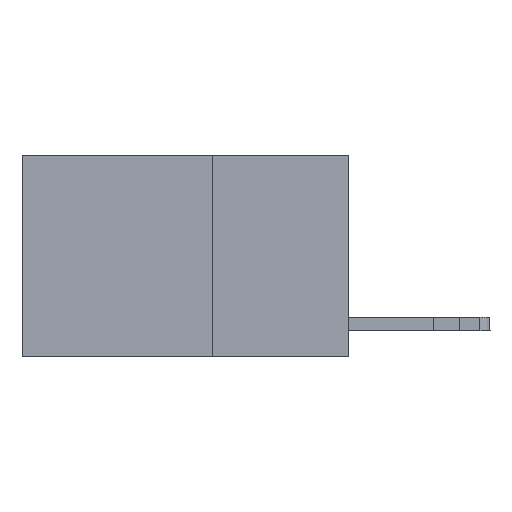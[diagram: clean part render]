
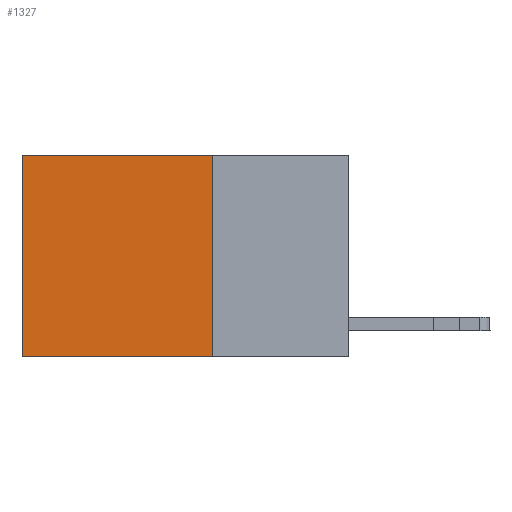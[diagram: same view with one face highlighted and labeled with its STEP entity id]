
A CAD part, left-side view. The second image highlights one B-rep face of the part: STEP entity #1327.
In plain terms, the highlighted planar face has unit normal (-1, 0, 0).
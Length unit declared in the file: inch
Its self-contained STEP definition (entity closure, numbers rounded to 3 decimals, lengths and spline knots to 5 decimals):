
#274 = VECTOR ( 'NONE', #15278, 39.37008 ) ;
#534 = VERTEX_POINT ( 'NONE', #18647 ) ;
#659 = VERTEX_POINT ( 'NONE', #11992 ) ;
#1327 = ADVANCED_FACE ( 'NONE', ( #2939 ), #8138, .F. ) ;
#2228 = EDGE_CURVE ( 'NONE', #659, #534, #5948, .T. ) ;
#2939 = FACE_OUTER_BOUND ( 'NONE', #16545, .T. ) ;
#2956 = EDGE_CURVE ( 'NONE', #12312, #534, #3242, .T. ) ;
#3242 = LINE ( 'NONE', #8800, #4995 ) ;
#4404 = EDGE_CURVE ( 'NONE', #12750, #659, #11387, .T. ) ;
#4995 = VECTOR ( 'NONE', #13891, 39.37008 ) ;
#5637 = ORIENTED_EDGE ( 'NONE', *, *, #4404, .T. ) ;
#5948 = LINE ( 'NONE', #21252, #7527 ) ;
#6313 = CARTESIAN_POINT ( 'NONE',  ( 0.2625, 0.25, 0. ) ) ;
#7310 = ORIENTED_EDGE ( 'NONE', *, *, #2228, .T. ) ;
#7527 = VECTOR ( 'NONE', #11985, 39.37008 ) ;
#8138 = PLANE ( 'NONE',  #18857 ) ;
#8800 = CARTESIAN_POINT ( 'NONE',  ( 0.2625, 0.25, -0.37 ) ) ;
#9334 = ORIENTED_EDGE ( 'NONE', *, *, #2956, .F. ) ;
#10310 = CARTESIAN_POINT ( 'NONE',  ( 0.2625, 0.25, 0. ) ) ;
#11387 = LINE ( 'NONE', #15049, #274 ) ;
#11985 = DIRECTION ( 'NONE',  ( 0., 0., -1. ) ) ;
#11992 = CARTESIAN_POINT ( 'NONE',  ( 0.2625, 0.6, 0. ) ) ;
#12312 = VERTEX_POINT ( 'NONE', #22286 ) ;
#12520 = EDGE_CURVE ( 'NONE', #12750, #12312, #22609, .T. ) ;
#12750 = VERTEX_POINT ( 'NONE', #18280 ) ;
#13239 = ORIENTED_EDGE ( 'NONE', *, *, #12520, .F. ) ;
#13891 = DIRECTION ( 'NONE',  ( 0., 1., 0. ) ) ;
#15049 = CARTESIAN_POINT ( 'NONE',  ( 0.2625, 0.25, 0. ) ) ;
#15278 = DIRECTION ( 'NONE',  ( 0., 1., 0. ) ) ;
#15410 = DIRECTION ( 'NONE',  ( 0., 0., -1. ) ) ;
#16545 = EDGE_LOOP ( 'NONE', ( #7310, #9334, #13239, #5637 ) ) ;
#17274 = DIRECTION ( 'NONE',  ( 0., 0., -1. ) ) ;
#18280 = CARTESIAN_POINT ( 'NONE',  ( 0.2625, 0.25, 0. ) ) ;
#18647 = CARTESIAN_POINT ( 'NONE',  ( 0.2625, 0.6, -0.37 ) ) ;
#18857 = AXIS2_PLACEMENT_3D ( 'NONE', #10310, #22805, #17274 ) ;
#21252 = CARTESIAN_POINT ( 'NONE',  ( 0.2625, 0.6, 0. ) ) ;
#21825 = VECTOR ( 'NONE', #15410, 39.37008 ) ;
#22286 = CARTESIAN_POINT ( 'NONE',  ( 0.2625, 0.25, -0.37 ) ) ;
#22609 = LINE ( 'NONE', #6313, #21825 ) ;
#22805 = DIRECTION ( 'NONE',  ( 1., 0., 0. ) ) ;
